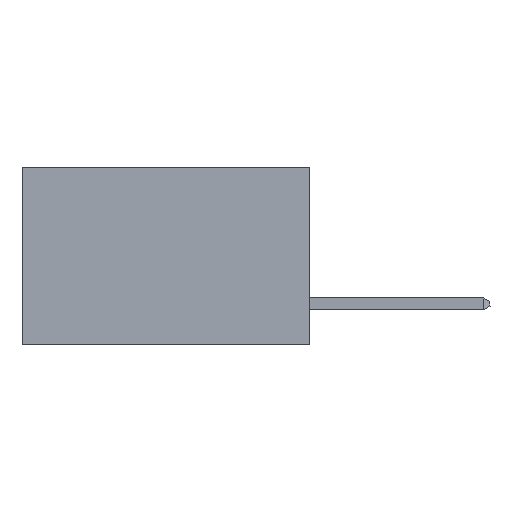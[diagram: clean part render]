
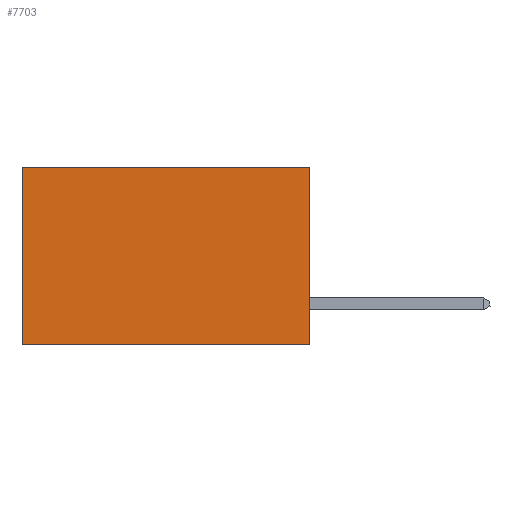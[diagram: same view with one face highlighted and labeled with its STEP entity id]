
A CAD part, left-side view. The second image highlights one B-rep face of the part: STEP entity #7703.
In plain terms, the highlighted planar face has unit normal (-1, 0, 0).
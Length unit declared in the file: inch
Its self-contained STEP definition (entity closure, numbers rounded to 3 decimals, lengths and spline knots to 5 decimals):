
#43 = EDGE_CURVE ( 'NONE', #7145, #4645, #2150, .T. ) ;
#530 = VERTEX_POINT ( 'NONE', #6053 ) ;
#1031 = ORIENTED_EDGE ( 'NONE', *, *, #43, .F. ) ;
#1323 = ORIENTED_EDGE ( 'NONE', *, *, #5072, .F. ) ;
#2016 = LINE ( 'NONE', #8621, #6045 ) ;
#2150 = LINE ( 'NONE', #2800, #10043 ) ;
#2407 = EDGE_LOOP ( 'NONE', ( #5691, #1323, #1031, #2775 ) ) ;
#2775 = ORIENTED_EDGE ( 'NONE', *, *, #7787, .T. ) ;
#2800 = CARTESIAN_POINT ( 'NONE',  ( 0.2875, 0., 0. ) ) ;
#3281 = VECTOR ( 'NONE', #3407, 39.37008 ) ;
#3407 = DIRECTION ( 'NONE',  ( 0., 1., 0. ) ) ;
#3637 = CARTESIAN_POINT ( 'NONE',  ( 0.2875, 0., 0. ) ) ;
#3817 = EDGE_CURVE ( 'NONE', #7647, #530, #2016, .T. ) ;
#4055 = DIRECTION ( 'NONE',  ( 0., 0., -1. ) ) ;
#4287 = CARTESIAN_POINT ( 'NONE',  ( 0.2875, 0.6, 0. ) ) ;
#4309 = DIRECTION ( 'NONE',  ( 0., 1., 0. ) ) ;
#4375 = CARTESIAN_POINT ( 'NONE',  ( 0.2875, 0., -0.37 ) ) ;
#4645 = VERTEX_POINT ( 'NONE', #5237 ) ;
#5072 = EDGE_CURVE ( 'NONE', #4645, #530, #8796, .T. ) ;
#5237 = CARTESIAN_POINT ( 'NONE',  ( 0.2875, 0., -0.37 ) ) ;
#5360 = DIRECTION ( 'NONE',  ( 1., 0., 0. ) ) ;
#5444 = LINE ( 'NONE', #3637, #3281 ) ;
#5691 = ORIENTED_EDGE ( 'NONE', *, *, #3817, .T. ) ;
#6026 = DIRECTION ( 'NONE',  ( 0., 0., -1. ) ) ;
#6045 = VECTOR ( 'NONE', #8636, 39.37008 ) ;
#6053 = CARTESIAN_POINT ( 'NONE',  ( 0.2875, 0.6, -0.37 ) ) ;
#6651 = VECTOR ( 'NONE', #4309, 39.37008 ) ;
#6713 = FACE_OUTER_BOUND ( 'NONE', #2407, .T. ) ;
#7145 = VERTEX_POINT ( 'NONE', #9604 ) ;
#7647 = VERTEX_POINT ( 'NONE', #4287 ) ;
#7703 = ADVANCED_FACE ( 'NONE', ( #6713 ), #8491, .F. ) ;
#7787 = EDGE_CURVE ( 'NONE', #7145, #7647, #5444, .T. ) ;
#8491 = PLANE ( 'NONE',  #9858 ) ;
#8621 = CARTESIAN_POINT ( 'NONE',  ( 0.2875, 0.6, 0. ) ) ;
#8636 = DIRECTION ( 'NONE',  ( 0., 0., -1. ) ) ;
#8796 = LINE ( 'NONE', #4375, #6651 ) ;
#9604 = CARTESIAN_POINT ( 'NONE',  ( 0.2875, 0., 0. ) ) ;
#9858 = AXIS2_PLACEMENT_3D ( 'NONE', #9994, #5360, #4055 ) ;
#9994 = CARTESIAN_POINT ( 'NONE',  ( 0.2875, 0., 0. ) ) ;
#10043 = VECTOR ( 'NONE', #6026, 39.37008 ) ;
